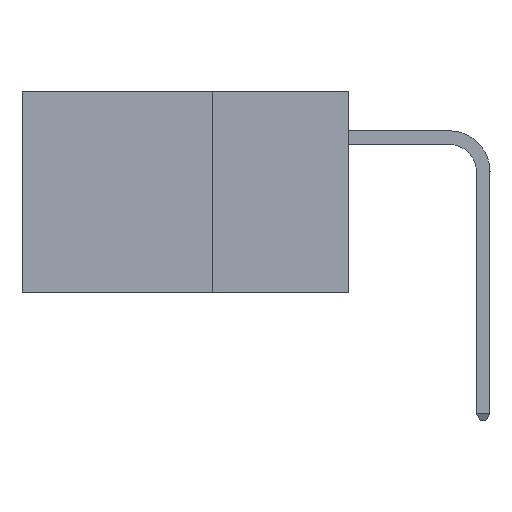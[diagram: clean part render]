
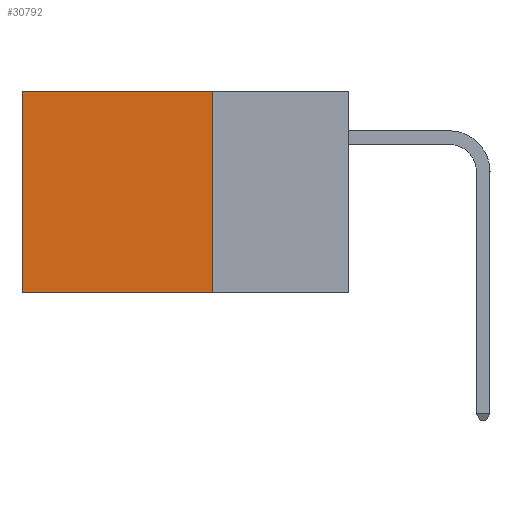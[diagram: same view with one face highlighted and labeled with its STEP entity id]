
A CAD part, left-side view. The second image highlights one B-rep face of the part: STEP entity #30792.
In plain terms, the highlighted planar face has unit normal (-1, 0, 0).
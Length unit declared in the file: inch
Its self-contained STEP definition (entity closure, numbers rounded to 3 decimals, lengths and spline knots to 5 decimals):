
#963 = CARTESIAN_POINT ( 'NONE',  ( 0.2875, 0.6, -0.37 ) ) ;
#982 = DIRECTION ( 'NONE',  ( 0., 1., 0. ) ) ;
#1678 = ORIENTED_EDGE ( 'NONE', *, *, #34725, .F. ) ;
#1802 = LINE ( 'NONE', #9246, #29713 ) ;
#2833 = ORIENTED_EDGE ( 'NONE', *, *, #11454, .F. ) ;
#2981 = ORIENTED_EDGE ( 'NONE', *, *, #10037, .T. ) ;
#4058 = VERTEX_POINT ( 'NONE', #31646 ) ;
#4961 = VERTEX_POINT ( 'NONE', #15138 ) ;
#5030 = LINE ( 'NONE', #5479, #20506 ) ;
#5479 = CARTESIAN_POINT ( 'NONE',  ( 0.2875, 0.25, 0. ) ) ;
#6907 = VECTOR ( 'NONE', #15507, 39.37008 ) ;
#9246 = CARTESIAN_POINT ( 'NONE',  ( 0.2875, 0.25, -0.37 ) ) ;
#9945 = CARTESIAN_POINT ( 'NONE',  ( 0.2875, 0.25, 0. ) ) ;
#10037 = EDGE_CURVE ( 'NONE', #4058, #33791, #14196, .T. ) ;
#11454 = EDGE_CURVE ( 'NONE', #4058, #4961, #5030, .T. ) ;
#13681 = DIRECTION ( 'NONE',  ( 0., 0., -1. ) ) ;
#14196 = LINE ( 'NONE', #9945, #6907 ) ;
#15138 = CARTESIAN_POINT ( 'NONE',  ( 0.2875, 0.25, -0.37 ) ) ;
#15507 = DIRECTION ( 'NONE',  ( 0., 1., 0. ) ) ;
#15776 = EDGE_CURVE ( 'NONE', #33791, #26142, #26761, .T. ) ;
#16456 = CARTESIAN_POINT ( 'NONE',  ( 0.2875, 0.25, 0. ) ) ;
#19143 = DIRECTION ( 'NONE',  ( 0., 0., -1. ) ) ;
#19464 = EDGE_LOOP ( 'NONE', ( #32884, #1678, #2833, #2981 ) ) ;
#19763 = CARTESIAN_POINT ( 'NONE',  ( 0.2875, 0.6, 0. ) ) ;
#20506 = VECTOR ( 'NONE', #13681, 39.37008 ) ;
#25923 = VECTOR ( 'NONE', #27416, 39.37008 ) ;
#26142 = VERTEX_POINT ( 'NONE', #963 ) ;
#26761 = LINE ( 'NONE', #29876, #25923 ) ;
#27002 = PLANE ( 'NONE',  #29295 ) ;
#27416 = DIRECTION ( 'NONE',  ( 0., 0., -1. ) ) ;
#29295 = AXIS2_PLACEMENT_3D ( 'NONE', #16456, #34613, #19143 ) ;
#29713 = VECTOR ( 'NONE', #982, 39.37008 ) ;
#29876 = CARTESIAN_POINT ( 'NONE',  ( 0.2875, 0.6, 0. ) ) ;
#29955 = FACE_OUTER_BOUND ( 'NONE', #19464, .T. ) ;
#30792 = ADVANCED_FACE ( 'NONE', ( #29955 ), #27002, .F. ) ;
#31646 = CARTESIAN_POINT ( 'NONE',  ( 0.2875, 0.25, 0. ) ) ;
#32884 = ORIENTED_EDGE ( 'NONE', *, *, #15776, .T. ) ;
#33791 = VERTEX_POINT ( 'NONE', #19763 ) ;
#34613 = DIRECTION ( 'NONE',  ( 1., 0., 0. ) ) ;
#34725 = EDGE_CURVE ( 'NONE', #4961, #26142, #1802, .T. ) ;
